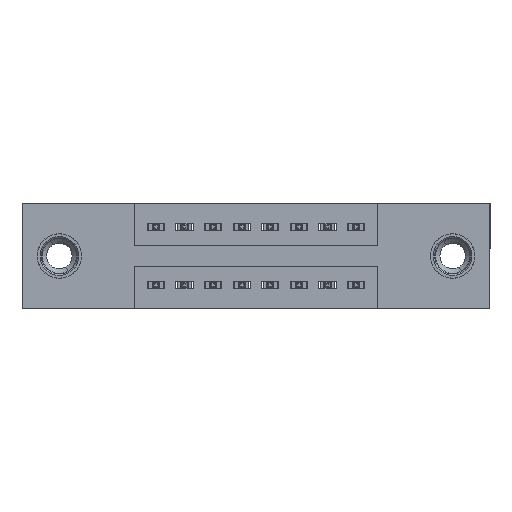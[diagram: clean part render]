
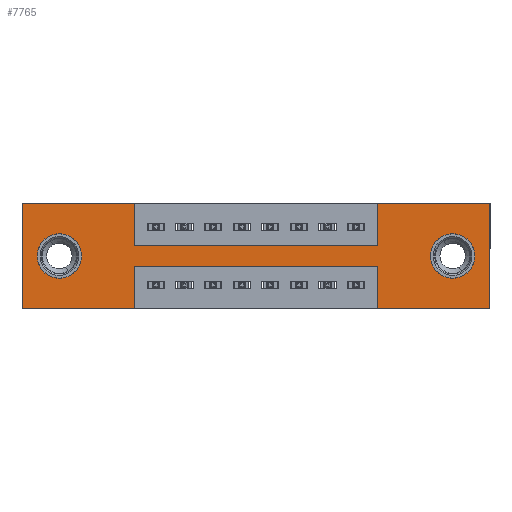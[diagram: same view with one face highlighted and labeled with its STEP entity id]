
A CAD part, front view. The second image highlights one B-rep face of the part: STEP entity #7765.
In plain terms, the highlighted planar face has unit normal (0, -1, 0).
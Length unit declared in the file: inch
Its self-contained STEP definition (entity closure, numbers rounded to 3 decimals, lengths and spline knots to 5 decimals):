
#49 = CARTESIAN_POINT ( 'NONE',  ( 0.3925, 0., -0.15 ) ) ;
#222 = VECTOR ( 'NONE', #15417, 39.37008 ) ;
#331 = CARTESIAN_POINT ( 'NONE',  ( 0., 0., 0. ) ) ;
#367 = ORIENTED_EDGE ( 'NONE', *, *, #12989, .F. ) ;
#496 = VERTEX_POINT ( 'NONE', #49 ) ;
#500 = CARTESIAN_POINT ( 'NONE',  ( 0.13, 0., -0.263 ) ) ;
#534 = CARTESIAN_POINT ( 'NONE',  ( 0.3925, 0., -0.37 ) ) ;
#648 = LINE ( 'NONE', #13919, #9024 ) ;
#683 = VECTOR ( 'NONE', #13506, 39.37008 ) ;
#708 = FACE_BOUND ( 'NONE', #2951, .T. ) ;
#758 = EDGE_CURVE ( 'NONE', #3410, #11498, #12870, .T. ) ;
#901 = EDGE_CURVE ( 'NONE', #496, #12291, #8677, .T. ) ;
#1374 = VECTOR ( 'NONE', #9035, 39.37008 ) ;
#1459 = VECTOR ( 'NONE', #10729, 39.37008 ) ;
#1532 = EDGE_CURVE ( 'NONE', #10439, #14934, #14923, .T. ) ;
#1788 = LINE ( 'NONE', #8865, #5506 ) ;
#1800 = ORIENTED_EDGE ( 'NONE', *, *, #11333, .T. ) ;
#1834 = EDGE_CURVE ( 'NONE', #9007, #4341, #11487, .T. ) ;
#2122 = DIRECTION ( 'NONE',  ( 0., -1., 0. ) ) ;
#2145 = EDGE_CURVE ( 'NONE', #10763, #496, #1788, .T. ) ;
#2266 = AXIS2_PLACEMENT_3D ( 'NONE', #11867, #14167, #14313 ) ;
#2541 = VERTEX_POINT ( 'NONE', #7493 ) ;
#2575 = VERTEX_POINT ( 'NONE', #8923 ) ;
#2583 = CARTESIAN_POINT ( 'NONE',  ( 1.2425, 0., 0. ) ) ;
#2638 = LINE ( 'NONE', #10125, #8257 ) ;
#2951 = EDGE_LOOP ( 'NONE', ( #1800, #12531 ) ) ;
#2978 = LINE ( 'NONE', #534, #1374 ) ;
#3030 = CARTESIAN_POINT ( 'NONE',  ( 0.3925, 0., -0.37 ) ) ;
#3272 = DIRECTION ( 'NONE',  ( 0., 1., 0. ) ) ;
#3398 = DIRECTION ( 'NONE',  ( 1., 0., 0. ) ) ;
#3410 = VERTEX_POINT ( 'NONE', #8867 ) ;
#3582 = EDGE_CURVE ( 'NONE', #11853, #9423, #5030, .T. ) ;
#3692 = ORIENTED_EDGE ( 'NONE', *, *, #4378, .F. ) ;
#3716 = ORIENTED_EDGE ( 'NONE', *, *, #1834, .F. ) ;
#4001 = VECTOR ( 'NONE', #4240, 39.37008 ) ;
#4092 = DIRECTION ( 'NONE',  ( 0., 0., -1. ) ) ;
#4240 = DIRECTION ( 'NONE',  ( -1., 0., 0. ) ) ;
#4298 = ORIENTED_EDGE ( 'NONE', *, *, #1532, .F. ) ;
#4341 = VERTEX_POINT ( 'NONE', #8828 ) ;
#4378 = EDGE_CURVE ( 'NONE', #4986, #2541, #11514, .T. ) ;
#4513 = AXIS2_PLACEMENT_3D ( 'NONE', #9545, #4761, #8285 ) ;
#4761 = DIRECTION ( 'NONE',  ( 0., 1., 0. ) ) ;
#4942 = ORIENTED_EDGE ( 'NONE', *, *, #5183, .T. ) ;
#4986 = VERTEX_POINT ( 'NONE', #10774 ) ;
#5030 = CIRCLE ( 'NONE', #2266, 0.078 ) ;
#5183 = EDGE_CURVE ( 'NONE', #9423, #11853, #5799, .T. ) ;
#5305 = PLANE ( 'NONE',  #10512 ) ;
#5420 = CARTESIAN_POINT ( 'NONE',  ( 0., 0., -0.37 ) ) ;
#5489 = DIRECTION ( 'NONE',  ( 0., 0., -1. ) ) ;
#5506 = VECTOR ( 'NONE', #6469, 39.37008 ) ;
#5541 = CARTESIAN_POINT ( 'NONE',  ( 1.2425, 0., -0.37 ) ) ;
#5578 = CARTESIAN_POINT ( 'NONE',  ( 1.635, 0., -0.37 ) ) ;
#5618 = EDGE_LOOP ( 'NONE', ( #8276, #3692, #13629, #7334, #4298, #13208, #367, #6701, #7317, #10377, #8443, #3716 ) ) ;
#5799 = CIRCLE ( 'NONE', #4513, 0.078 ) ;
#6282 = EDGE_CURVE ( 'NONE', #12276, #4986, #6849, .T. ) ;
#6415 = DIRECTION ( 'NONE',  ( 0., 1., 0. ) ) ;
#6469 = DIRECTION ( 'NONE',  ( 0., 0., -1. ) ) ;
#6473 = CARTESIAN_POINT ( 'NONE',  ( 0.13, 0., -0.107 ) ) ;
#6701 = ORIENTED_EDGE ( 'NONE', *, *, #901, .F. ) ;
#6849 = LINE ( 'NONE', #11933, #1459 ) ;
#7067 = DIRECTION ( 'NONE',  ( 0., 0., -1. ) ) ;
#7204 = LINE ( 'NONE', #2583, #10024 ) ;
#7317 = ORIENTED_EDGE ( 'NONE', *, *, #2145, .F. ) ;
#7334 = ORIENTED_EDGE ( 'NONE', *, *, #8996, .F. ) ;
#7493 = CARTESIAN_POINT ( 'NONE',  ( 0.3925, 0., -0.22 ) ) ;
#7500 = DIRECTION ( 'NONE',  ( 0., 0., 1. ) ) ;
#7759 = VECTOR ( 'NONE', #14487, 39.37008 ) ;
#7765 = ADVANCED_FACE ( 'NONE', ( #708, #14867, #10017 ), #5305, .T. ) ;
#7944 = CARTESIAN_POINT ( 'NONE',  ( 1.2425, 0., -0.15 ) ) ;
#7979 = VECTOR ( 'NONE', #3398, 39.37008 ) ;
#8074 = CARTESIAN_POINT ( 'NONE',  ( 1.505, 0., -0.107 ) ) ;
#8186 = CARTESIAN_POINT ( 'NONE',  ( 0., 0., 0. ) ) ;
#8257 = VECTOR ( 'NONE', #7500, 39.37008 ) ;
#8276 = ORIENTED_EDGE ( 'NONE', *, *, #10250, .F. ) ;
#8285 = DIRECTION ( 'NONE',  ( 0., 0., 1. ) ) ;
#8443 = ORIENTED_EDGE ( 'NONE', *, *, #8913, .F. ) ;
#8677 = LINE ( 'NONE', #11864, #683 ) ;
#8805 = CARTESIAN_POINT ( 'NONE',  ( 1.505, 0., -0.185 ) ) ;
#8828 = CARTESIAN_POINT ( 'NONE',  ( 0., 0., -0.37 ) ) ;
#8865 = CARTESIAN_POINT ( 'NONE',  ( 0.3925, 0., 0. ) ) ;
#8867 = CARTESIAN_POINT ( 'NONE',  ( 1.505, 0., -0.263 ) ) ;
#8913 = EDGE_CURVE ( 'NONE', #4341, #15491, #2638, .T. ) ;
#8923 = CARTESIAN_POINT ( 'NONE',  ( 1.2425, 0., 0. ) ) ;
#8957 = DIRECTION ( 'NONE',  ( 0., 0., -1. ) ) ;
#8996 = EDGE_CURVE ( 'NONE', #14934, #12276, #648, .T. ) ;
#9007 = VERTEX_POINT ( 'NONE', #3030 ) ;
#9024 = VECTOR ( 'NONE', #11532, 39.37008 ) ;
#9035 = DIRECTION ( 'NONE',  ( 0., 0., -1. ) ) ;
#9253 = CIRCLE ( 'NONE', #12571, 0.078 ) ;
#9423 = VERTEX_POINT ( 'NONE', #500 ) ;
#9529 = LINE ( 'NONE', #8186, #7979 ) ;
#9545 = CARTESIAN_POINT ( 'NONE',  ( 0.13, 0., -0.185 ) ) ;
#9934 = EDGE_LOOP ( 'NONE', ( #13277, #4942 ) ) ;
#10017 = FACE_OUTER_BOUND ( 'NONE', #5618, .T. ) ;
#10024 = VECTOR ( 'NONE', #12048, 39.37008 ) ;
#10125 = CARTESIAN_POINT ( 'NONE',  ( 0., 0., 0. ) ) ;
#10250 = EDGE_CURVE ( 'NONE', #2541, #9007, #2978, .T. ) ;
#10377 = ORIENTED_EDGE ( 'NONE', *, *, #10719, .F. ) ;
#10439 = VERTEX_POINT ( 'NONE', #10986 ) ;
#10512 = AXIS2_PLACEMENT_3D ( 'NONE', #15019, #2122, #7067 ) ;
#10719 = EDGE_CURVE ( 'NONE', #15491, #10763, #9529, .T. ) ;
#10729 = DIRECTION ( 'NONE',  ( 0., 0., 1. ) ) ;
#10763 = VERTEX_POINT ( 'NONE', #14787 ) ;
#10774 = CARTESIAN_POINT ( 'NONE',  ( 1.2425, 0., -0.22 ) ) ;
#10986 = CARTESIAN_POINT ( 'NONE',  ( 1.635, 0., 0. ) ) ;
#11333 = EDGE_CURVE ( 'NONE', #11498, #3410, #9253, .T. ) ;
#11367 = VECTOR ( 'NONE', #8957, 39.37008 ) ;
#11487 = LINE ( 'NONE', #5420, #4001 ) ;
#11498 = VERTEX_POINT ( 'NONE', #8074 ) ;
#11514 = LINE ( 'NONE', #15183, #222 ) ;
#11532 = DIRECTION ( 'NONE',  ( -1., 0., 0. ) ) ;
#11853 = VERTEX_POINT ( 'NONE', #6473 ) ;
#11864 = CARTESIAN_POINT ( 'NONE',  ( 0.3925, 0., -0.15 ) ) ;
#11867 = CARTESIAN_POINT ( 'NONE',  ( 0.13, 0., -0.185 ) ) ;
#11933 = CARTESIAN_POINT ( 'NONE',  ( 1.2425, 0., -0.37 ) ) ;
#11957 = CARTESIAN_POINT ( 'NONE',  ( 0., 0., 0. ) ) ;
#12048 = DIRECTION ( 'NONE',  ( 0., 0., 1. ) ) ;
#12276 = VERTEX_POINT ( 'NONE', #5541 ) ;
#12291 = VERTEX_POINT ( 'NONE', #7944 ) ;
#12384 = CARTESIAN_POINT ( 'NONE',  ( 1.635, 0., 0. ) ) ;
#12531 = ORIENTED_EDGE ( 'NONE', *, *, #758, .T. ) ;
#12571 = AXIS2_PLACEMENT_3D ( 'NONE', #8805, #6415, #4092 ) ;
#12870 = CIRCLE ( 'NONE', #13115, 0.078 ) ;
#12989 = EDGE_CURVE ( 'NONE', #12291, #2575, #7204, .T. ) ;
#13115 = AXIS2_PLACEMENT_3D ( 'NONE', #14163, #3272, #5489 ) ;
#13141 = LINE ( 'NONE', #11957, #7759 ) ;
#13208 = ORIENTED_EDGE ( 'NONE', *, *, #13997, .F. ) ;
#13277 = ORIENTED_EDGE ( 'NONE', *, *, #3582, .T. ) ;
#13506 = DIRECTION ( 'NONE',  ( 1., 0., 0. ) ) ;
#13629 = ORIENTED_EDGE ( 'NONE', *, *, #6282, .F. ) ;
#13919 = CARTESIAN_POINT ( 'NONE',  ( 0., 0., -0.37 ) ) ;
#13997 = EDGE_CURVE ( 'NONE', #2575, #10439, #13141, .T. ) ;
#14163 = CARTESIAN_POINT ( 'NONE',  ( 1.505, 0., -0.185 ) ) ;
#14167 = DIRECTION ( 'NONE',  ( 0., 1., 0. ) ) ;
#14313 = DIRECTION ( 'NONE',  ( 0., 0., 1. ) ) ;
#14487 = DIRECTION ( 'NONE',  ( 1., 0., 0. ) ) ;
#14787 = CARTESIAN_POINT ( 'NONE',  ( 0.3925, 0., 0. ) ) ;
#14867 = FACE_BOUND ( 'NONE', #9934, .T. ) ;
#14923 = LINE ( 'NONE', #12384, #11367 ) ;
#14934 = VERTEX_POINT ( 'NONE', #5578 ) ;
#15019 = CARTESIAN_POINT ( 'NONE',  ( 0., 0., -0.37 ) ) ;
#15183 = CARTESIAN_POINT ( 'NONE',  ( 0.3925, 0., -0.22 ) ) ;
#15417 = DIRECTION ( 'NONE',  ( -1., 0., 0. ) ) ;
#15491 = VERTEX_POINT ( 'NONE', #331 ) ;
